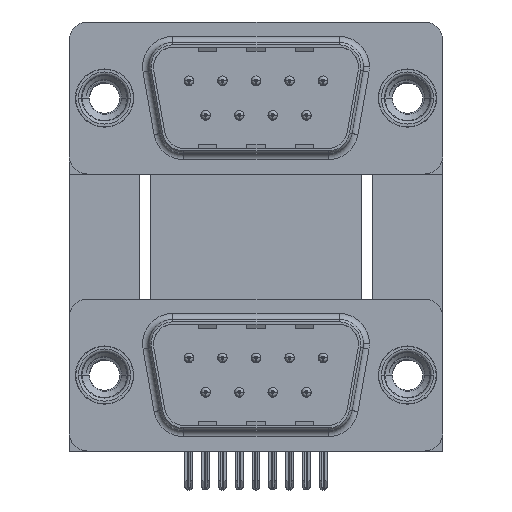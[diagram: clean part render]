
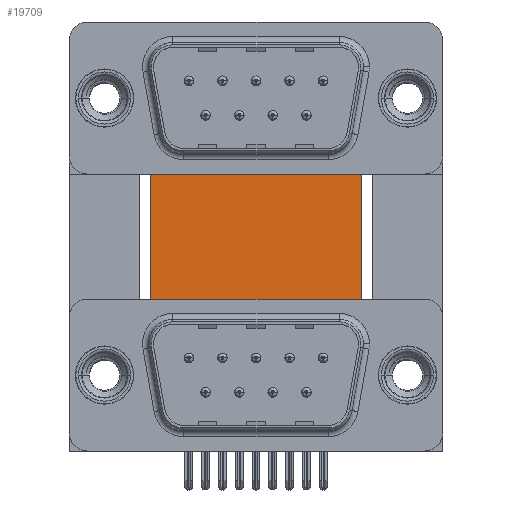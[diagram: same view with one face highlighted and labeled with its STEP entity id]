
A CAD part, top view. The second image highlights one B-rep face of the part: STEP entity #19709.
In plain terms, the highlighted planar face has unit normal (0, 0, 1).
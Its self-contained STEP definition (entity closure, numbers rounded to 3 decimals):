
#436 = DIRECTION ( 'NONE',  ( 1., 0., 0. ) ) ;
#743 = DIRECTION ( 'NONE',  ( 1., 0., 0. ) ) ;
#785 = EDGE_CURVE ( 'NONE', #27268, #16266, #7412, .T. ) ;
#819 = DIRECTION ( 'NONE',  ( 0., -1., 0. ) ) ;
#874 = ORIENTED_EDGE ( 'NONE', *, *, #23207, .F. ) ;
#1413 = DIRECTION ( 'NONE',  ( 1., 0., 0. ) ) ;
#1849 = CARTESIAN_POINT ( 'NONE',  ( 22.59, -4.635, -12. ) ) ;
#2397 = DIRECTION ( 'NONE',  ( 1., 0., 0. ) ) ;
#2722 = LINE ( 'NONE', #11417, #19874 ) ;
#3082 = VECTOR ( 'NONE', #22825, 1000. ) ;
#3147 = CARTESIAN_POINT ( 'NONE',  ( 3.79, 16.585, -12. ) ) ;
#5319 = VERTEX_POINT ( 'NONE', #24173 ) ;
#5361 = CARTESIAN_POINT ( 'NONE',  ( 3.79, -0.735, -12. ) ) ;
#5523 = VERTEX_POINT ( 'NONE', #8010 ) ;
#5807 = DIRECTION ( 'NONE',  ( 0., 0., -1. ) ) ;
#5871 = EDGE_CURVE ( 'NONE', #5523, #5319, #22672, .T. ) ;
#6365 = CARTESIAN_POINT ( 'NONE',  ( 2.9, -4.635, -12. ) ) ;
#6549 = LINE ( 'NONE', #15258, #7414 ) ;
#7102 = VERTEX_POINT ( 'NONE', #17576 ) ;
#7184 = EDGE_CURVE ( 'NONE', #7102, #16918, #11286, .T. ) ;
#7264 = EDGE_CURVE ( 'NONE', #16374, #27268, #2722, .T. ) ;
#7412 = LINE ( 'NONE', #18415, #21619 ) ;
#7414 = VECTOR ( 'NONE', #2397, 1000. ) ;
#7729 = CARTESIAN_POINT ( 'NONE',  ( 22.09, -4.635, -12. ) ) ;
#7791 = CARTESIAN_POINT ( 'NONE',  ( 2.9, -3.735, -12. ) ) ;
#8010 = CARTESIAN_POINT ( 'NONE',  ( 22.09, -3.735, -12. ) ) ;
#8101 = EDGE_CURVE ( 'NONE', #7102, #16374, #17853, .T. ) ;
#8108 = LINE ( 'NONE', #14104, #3082 ) ;
#8170 = DIRECTION ( 'NONE',  ( -0.336, 0.942, 0. ) ) ;
#8547 = VECTOR ( 'NONE', #743, 1000. ) ;
#9202 = VERTEX_POINT ( 'NONE', #15319 ) ;
#9951 = DIRECTION ( 'NONE',  ( -1., 0., 0. ) ) ;
#9983 = EDGE_CURVE ( 'NONE', #9202, #5523, #6549, .T. ) ;
#11286 = LINE ( 'NONE', #13849, #25816 ) ;
#11417 = CARTESIAN_POINT ( 'NONE',  ( 2.4, -4.635, -12. ) ) ;
#11520 = VECTOR ( 'NONE', #819, 1000. ) ;
#11653 = VECTOR ( 'NONE', #8170, 1000. ) ;
#11832 = VERTEX_POINT ( 'NONE', #1849 ) ;
#12046 = EDGE_LOOP ( 'NONE', ( #19611, #15008, #25440, #26302, #874, #23366, #14182, #15259, #16960, #12352 ) ) ;
#12213 = LINE ( 'NONE', #7791, #13840 ) ;
#12338 = CARTESIAN_POINT ( 'NONE',  ( 21.2, 16.585, -12. ) ) ;
#12352 = ORIENTED_EDGE ( 'NONE', *, *, #24866, .T. ) ;
#12667 = CARTESIAN_POINT ( 'NONE',  ( 2.4, -4.635, -12. ) ) ;
#13742 = VERTEX_POINT ( 'NONE', #27002 ) ;
#13840 = VECTOR ( 'NONE', #14081, 1000. ) ;
#13849 = CARTESIAN_POINT ( 'NONE',  ( 3.79, 16.585, -12. ) ) ;
#14081 = DIRECTION ( 'NONE',  ( 0., 1., 0. ) ) ;
#14104 = CARTESIAN_POINT ( 'NONE',  ( 21.2, 16.585, -12. ) ) ;
#14182 = ORIENTED_EDGE ( 'NONE', *, *, #8101, .T. ) ;
#14259 = DIRECTION ( 'NONE',  ( -0.336, -0.942, 0. ) ) ;
#15008 = ORIENTED_EDGE ( 'NONE', *, *, #5871, .T. ) ;
#15258 = CARTESIAN_POINT ( 'NONE',  ( 3.79, -3.735, -12. ) ) ;
#15259 = ORIENTED_EDGE ( 'NONE', *, *, #7264, .T. ) ;
#15319 = CARTESIAN_POINT ( 'NONE',  ( 2.9, -3.735, -12. ) ) ;
#15951 = CARTESIAN_POINT ( 'NONE',  ( 22.09, -3.735, -12. ) ) ;
#16266 = VERTEX_POINT ( 'NONE', #6365 ) ;
#16294 = LINE ( 'NONE', #7729, #8547 ) ;
#16374 = VERTEX_POINT ( 'NONE', #5361 ) ;
#16789 = FACE_OUTER_BOUND ( 'NONE', #12046, .T. ) ;
#16918 = VERTEX_POINT ( 'NONE', #12338 ) ;
#16960 = ORIENTED_EDGE ( 'NONE', *, *, #785, .T. ) ;
#17070 = VECTOR ( 'NONE', #20292, 1000. ) ;
#17576 = CARTESIAN_POINT ( 'NONE',  ( 3.79, 16.585, -12. ) ) ;
#17853 = LINE ( 'NONE', #3147, #17070 ) ;
#18380 = EDGE_CURVE ( 'NONE', #11832, #13742, #18750, .T. ) ;
#18415 = CARTESIAN_POINT ( 'NONE',  ( 2.9, -4.635, -12. ) ) ;
#18750 = LINE ( 'NONE', #27461, #11653 ) ;
#19611 = ORIENTED_EDGE ( 'NONE', *, *, #9983, .T. ) ;
#19709 = ADVANCED_FACE ( 'NONE', ( #16789 ), #27503, .F. ) ;
#19874 = VECTOR ( 'NONE', #14259, 1000. ) ;
#19935 = EDGE_CURVE ( 'NONE', #5319, #11832, #16294, .T. ) ;
#20292 = DIRECTION ( 'NONE',  ( 0., -1., 0. ) ) ;
#20394 = AXIS2_PLACEMENT_3D ( 'NONE', #25510, #5807, #9951 ) ;
#21619 = VECTOR ( 'NONE', #1413, 1000. ) ;
#22672 = LINE ( 'NONE', #15951, #11520 ) ;
#22825 = DIRECTION ( 'NONE',  ( 0., -1., 0. ) ) ;
#23207 = EDGE_CURVE ( 'NONE', #16918, #13742, #8108, .T. ) ;
#23366 = ORIENTED_EDGE ( 'NONE', *, *, #7184, .F. ) ;
#24173 = CARTESIAN_POINT ( 'NONE',  ( 22.09, -4.635, -12. ) ) ;
#24866 = EDGE_CURVE ( 'NONE', #16266, #9202, #12213, .T. ) ;
#25440 = ORIENTED_EDGE ( 'NONE', *, *, #19935, .T. ) ;
#25510 = CARTESIAN_POINT ( 'NONE',  ( 3.79, 16.585, -12. ) ) ;
#25816 = VECTOR ( 'NONE', #436, 1000. ) ;
#26302 = ORIENTED_EDGE ( 'NONE', *, *, #18380, .T. ) ;
#27002 = CARTESIAN_POINT ( 'NONE',  ( 21.2, -0.735, -12. ) ) ;
#27268 = VERTEX_POINT ( 'NONE', #12667 ) ;
#27461 = CARTESIAN_POINT ( 'NONE',  ( 22.59, -4.635, -12. ) ) ;
#27503 = PLANE ( 'NONE',  #20394 ) ;
